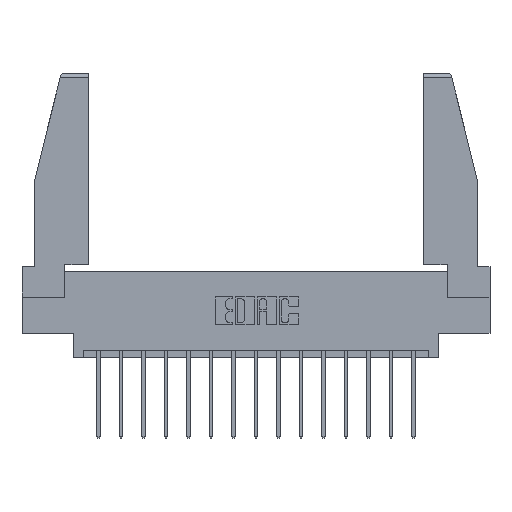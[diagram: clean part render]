
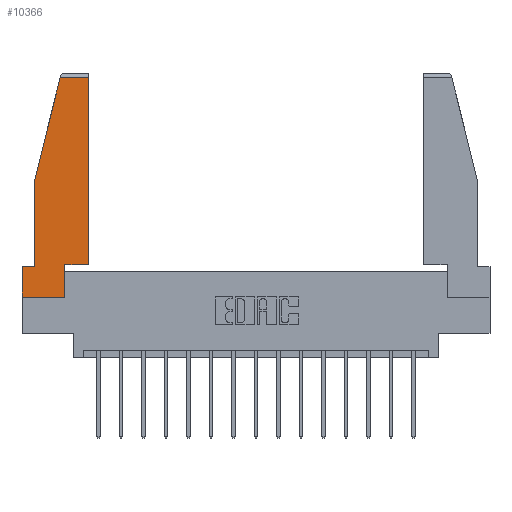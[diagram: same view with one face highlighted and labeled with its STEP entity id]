
A CAD part, top view. The second image highlights one B-rep face of the part: STEP entity #10366.
In plain terms, the highlighted planar face has unit normal (0, 0, 1).
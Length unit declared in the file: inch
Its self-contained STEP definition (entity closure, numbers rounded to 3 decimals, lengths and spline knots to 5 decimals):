
#629 = EDGE_CURVE ( 'NONE', #9857, #9917, #16951, .T. ) ;
#991 = DIRECTION ( 'NONE',  ( 0., -1., 0. ) ) ;
#2137 = ORIENTED_EDGE ( 'NONE', *, *, #6544, .T. ) ;
#2383 = ORIENTED_EDGE ( 'NONE', *, *, #17256, .T. ) ;
#2516 = CARTESIAN_POINT ( 'NONE',  ( 0.297, 0., 0. ) ) ;
#3085 = PLANE ( 'NONE',  #6792 ) ;
#3119 = VERTEX_POINT ( 'NONE', #13523 ) ;
#3662 = VECTOR ( 'NONE', #13356, 39.37008 ) ;
#3722 = CARTESIAN_POINT ( 'NONE',  ( 0., 0., 0. ) ) ;
#3787 = VECTOR ( 'NONE', #16730, 39.37008 ) ;
#4025 = VERTEX_POINT ( 'NONE', #17052 ) ;
#4066 = VERTEX_POINT ( 'NONE', #8911 ) ;
#4438 = DIRECTION ( 'NONE',  ( -1., 0., 0. ) ) ;
#4447 = CARTESIAN_POINT ( 'NONE',  ( 0.461, 0.223, 0. ) ) ;
#4651 = CARTESIAN_POINT ( 'NONE',  ( 0., 0., 0. ) ) ;
#4704 = DIRECTION ( 'NONE',  ( 0., 0., 1. ) ) ;
#5311 = CARTESIAN_POINT ( 'NONE',  ( 0.461, 1.52, 0. ) ) ;
#5869 = DIRECTION ( 'NONE',  ( 1., 0., 0. ) ) ;
#6343 = ORIENTED_EDGE ( 'NONE', *, *, #17387, .T. ) ;
#6452 = CARTESIAN_POINT ( 'NONE',  ( 0., 0.21, 0. ) ) ;
#6544 = EDGE_CURVE ( 'NONE', #17227, #3119, #13283, .T. ) ;
#6792 = AXIS2_PLACEMENT_3D ( 'NONE', #4651, #4704, #5869 ) ;
#7514 = ORIENTED_EDGE ( 'NONE', *, *, #12613, .T. ) ;
#7618 = VERTEX_POINT ( 'NONE', #14529 ) ;
#8499 = DIRECTION ( 'NONE',  ( 0., 1., 0. ) ) ;
#8642 = LINE ( 'NONE', #6452, #3662 ) ;
#8735 = DIRECTION ( 'NONE',  ( 1., 0., 0. ) ) ;
#8880 = EDGE_CURVE ( 'NONE', #9917, #17227, #11658, .T. ) ;
#8911 = CARTESIAN_POINT ( 'NONE',  ( 0.297, 0.223, 0. ) ) ;
#9246 = VECTOR ( 'NONE', #10612, 39.37008 ) ;
#9857 = VERTEX_POINT ( 'NONE', #17018 ) ;
#9917 = VERTEX_POINT ( 'NONE', #10575 ) ;
#9995 = DIRECTION ( 'NONE',  ( -0.239, -0.971, 0. ) ) ;
#10224 = LINE ( 'NONE', #12865, #13262 ) ;
#10366 = ADVANCED_FACE ( 'NONE', ( #16798 ), #3085, .T. ) ;
#10575 = CARTESIAN_POINT ( 'NONE',  ( 0.086, 0.8, 0. ) ) ;
#10612 = DIRECTION ( 'NONE',  ( 0., 1., 0. ) ) ;
#10638 = EDGE_CURVE ( 'NONE', #3119, #16941, #8642, .T. ) ;
#10880 = EDGE_LOOP ( 'NONE', ( #16452, #6343, #14712, #15447, #2137, #14974, #7514, #11896, #2383 ) ) ;
#11433 = CARTESIAN_POINT ( 'NONE',  ( 0., 1.52, 0. ) ) ;
#11535 = LINE ( 'NONE', #11433, #3787 ) ;
#11575 = VECTOR ( 'NONE', #9995, 39.37008 ) ;
#11637 = EDGE_CURVE ( 'NONE', #4025, #4066, #13543, .T. ) ;
#11658 = LINE ( 'NONE', #17283, #17235 ) ;
#11688 = DIRECTION ( 'NONE',  ( 1., 0., 0. ) ) ;
#11896 = ORIENTED_EDGE ( 'NONE', *, *, #11637, .T. ) ;
#12613 = EDGE_CURVE ( 'NONE', #16941, #4025, #17464, .T. ) ;
#12634 = LINE ( 'NONE', #4447, #13492 ) ;
#12865 = CARTESIAN_POINT ( 'NONE',  ( 0.297, 0.223, 0. ) ) ;
#12976 = VECTOR ( 'NONE', #11688, 39.37008 ) ;
#13262 = VECTOR ( 'NONE', #8735, 39.37008 ) ;
#13283 = LINE ( 'NONE', #13997, #16929 ) ;
#13356 = DIRECTION ( 'NONE',  ( 0., -1., 0. ) ) ;
#13492 = VECTOR ( 'NONE', #8499, 39.37008 ) ;
#13523 = CARTESIAN_POINT ( 'NONE',  ( 0., 0.21, 0. ) ) ;
#13543 = LINE ( 'NONE', #2516, #9246 ) ;
#13954 = VERTEX_POINT ( 'NONE', #5311 ) ;
#13997 = CARTESIAN_POINT ( 'NONE',  ( 0., 0.21, 0. ) ) ;
#14100 = CARTESIAN_POINT ( 'NONE',  ( 0.271, 1.55, 0. ) ) ;
#14529 = CARTESIAN_POINT ( 'NONE',  ( 0.461, 0.223, 0. ) ) ;
#14712 = ORIENTED_EDGE ( 'NONE', *, *, #629, .T. ) ;
#14974 = ORIENTED_EDGE ( 'NONE', *, *, #10638, .T. ) ;
#15447 = ORIENTED_EDGE ( 'NONE', *, *, #8880, .T. ) ;
#15529 = CARTESIAN_POINT ( 'NONE',  ( 0.086, 0.21, 0. ) ) ;
#15791 = CARTESIAN_POINT ( 'NONE',  ( 0., 0., 0. ) ) ;
#16452 = ORIENTED_EDGE ( 'NONE', *, *, #17057, .T. ) ;
#16730 = DIRECTION ( 'NONE',  ( -1., 0., 0. ) ) ;
#16798 = FACE_OUTER_BOUND ( 'NONE', #10880, .T. ) ;
#16929 = VECTOR ( 'NONE', #4438, 39.37008 ) ;
#16941 = VERTEX_POINT ( 'NONE', #3722 ) ;
#16951 = LINE ( 'NONE', #14100, #11575 ) ;
#17018 = CARTESIAN_POINT ( 'NONE',  ( 0.2636, 1.52, 0. ) ) ;
#17052 = CARTESIAN_POINT ( 'NONE',  ( 0.297, 0., 0. ) ) ;
#17057 = EDGE_CURVE ( 'NONE', #7618, #13954, #12634, .T. ) ;
#17227 = VERTEX_POINT ( 'NONE', #15529 ) ;
#17235 = VECTOR ( 'NONE', #991, 39.37008 ) ;
#17256 = EDGE_CURVE ( 'NONE', #4066, #7618, #10224, .T. ) ;
#17283 = CARTESIAN_POINT ( 'NONE',  ( 0.086, 0.8, 0. ) ) ;
#17387 = EDGE_CURVE ( 'NONE', #13954, #9857, #11535, .T. ) ;
#17464 = LINE ( 'NONE', #15791, #12976 ) ;
